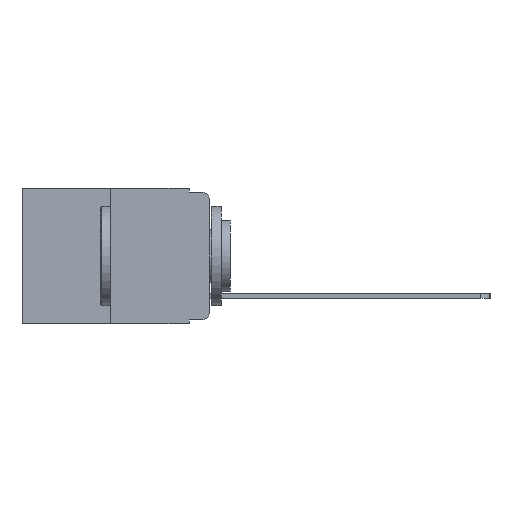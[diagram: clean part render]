
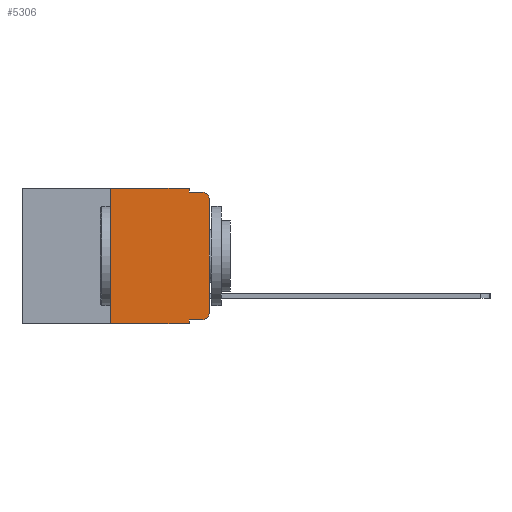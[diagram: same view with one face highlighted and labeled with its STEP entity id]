
A CAD part, left-side view. The second image highlights one B-rep face of the part: STEP entity #5306.
In plain terms, the highlighted planar face has unit normal (-1, 0, 0).
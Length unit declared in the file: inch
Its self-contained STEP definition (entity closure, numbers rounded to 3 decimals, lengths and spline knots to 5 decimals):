
#156 = CARTESIAN_POINT ( 'NONE',  ( 0., 0.051, 0. ) ) ;
#207 = VECTOR ( 'NONE', #7608, 39.37008 ) ;
#285 = CARTESIAN_POINT ( 'NONE',  ( 0., 0., 0. ) ) ;
#701 = CARTESIAN_POINT ( 'NONE',  ( 0., 0.051, -0.333 ) ) ;
#1088 = EDGE_CURVE ( 'NONE', #9467, #4476, #3043, .T. ) ;
#1211 = CARTESIAN_POINT ( 'NONE',  ( 0., 0.02, -0.01 ) ) ;
#1684 = CARTESIAN_POINT ( 'NONE',  ( 0., 0., -0.03 ) ) ;
#1837 = EDGE_CURVE ( 'NONE', #7003, #9919, #7429, .T. ) ;
#2026 = ORIENTED_EDGE ( 'NONE', *, *, #10799, .T. ) ;
#2175 = CARTESIAN_POINT ( 'NONE',  ( 0., 0.051, -0.01 ) ) ;
#2226 = DIRECTION ( 'NONE',  ( 0., 0., 1. ) ) ;
#2254 = DIRECTION ( 'NONE',  ( 0., 0., -1. ) ) ;
#2274 = DIRECTION ( 'NONE',  ( -1., 0., 0. ) ) ;
#2369 = VERTEX_POINT ( 'NONE', #5458 ) ;
#2558 = VECTOR ( 'NONE', #2886, 39.37008 ) ;
#2673 = LINE ( 'NONE', #2175, #9998 ) ;
#2846 = LINE ( 'NONE', #2920, #8355 ) ;
#2886 = DIRECTION ( 'NONE',  ( 0., -1., 0. ) ) ;
#2920 = CARTESIAN_POINT ( 'NONE',  ( 0., 0.051, -0.333 ) ) ;
#3043 = LINE ( 'NONE', #7490, #207 ) ;
#3110 = CARTESIAN_POINT ( 'NONE',  ( 0., 0.051, 0. ) ) ;
#3234 = EDGE_CURVE ( 'NONE', #5201, #7003, #6945, .T. ) ;
#3285 = CARTESIAN_POINT ( 'NONE',  ( 0., 0.25, 0. ) ) ;
#3453 = EDGE_CURVE ( 'NONE', #9909, #11802, #5152, .T. ) ;
#3486 = AXIS2_PLACEMENT_3D ( 'NONE', #8108, #2274, #2254 ) ;
#3503 = AXIS2_PLACEMENT_3D ( 'NONE', #9699, #10596, #6112 ) ;
#3666 = VERTEX_POINT ( 'NONE', #701 ) ;
#3677 = VERTEX_POINT ( 'NONE', #1211 ) ;
#3791 = PLANE ( 'NONE',  #3503 ) ;
#3971 = DIRECTION ( 'NONE',  ( 0., -1., 0. ) ) ;
#4102 = EDGE_LOOP ( 'NONE', ( #4177, #6776, #9177, #11504, #4493, #7070, #2026, #4822, #7376, #12063 ) ) ;
#4166 = LINE ( 'NONE', #156, #6481 ) ;
#4177 = ORIENTED_EDGE ( 'NONE', *, *, #1837, .T. ) ;
#4402 = EDGE_CURVE ( 'NONE', #9919, #3677, #12333, .T. ) ;
#4476 = VERTEX_POINT ( 'NONE', #8249 ) ;
#4493 = ORIENTED_EDGE ( 'NONE', *, *, #10351, .F. ) ;
#4822 = ORIENTED_EDGE ( 'NONE', *, *, #11854, .F. ) ;
#5036 = VECTOR ( 'NONE', #6316, 39.37008 ) ;
#5152 = LINE ( 'NONE', #10965, #9736 ) ;
#5201 = VERTEX_POINT ( 'NONE', #8906 ) ;
#5306 = ADVANCED_FACE ( 'NONE', ( #5813 ), #3791, .F. ) ;
#5458 = CARTESIAN_POINT ( 'NONE',  ( 0., 0.051, -0.343 ) ) ;
#5636 = LINE ( 'NONE', #5984, #2558 ) ;
#5813 = FACE_OUTER_BOUND ( 'NONE', #4102, .T. ) ;
#5984 = CARTESIAN_POINT ( 'NONE',  ( 0., 0.473, -0.343 ) ) ;
#6112 = DIRECTION ( 'NONE',  ( 0., 0., -1. ) ) ;
#6316 = DIRECTION ( 'NONE',  ( 0., -1., 0. ) ) ;
#6481 = VECTOR ( 'NONE', #8216, 39.37008 ) ;
#6776 = ORIENTED_EDGE ( 'NONE', *, *, #4402, .T. ) ;
#6945 = CIRCLE ( 'NONE', #3486, 0.02 ) ;
#7003 = VERTEX_POINT ( 'NONE', #7878 ) ;
#7070 = ORIENTED_EDGE ( 'NONE', *, *, #3453, .F. ) ;
#7376 = ORIENTED_EDGE ( 'NONE', *, *, #11530, .T. ) ;
#7429 = LINE ( 'NONE', #285, #9229 ) ;
#7490 = CARTESIAN_POINT ( 'NONE',  ( 0., 0.051, 0. ) ) ;
#7608 = DIRECTION ( 'NONE',  ( 0., 0., -1. ) ) ;
#7669 = CARTESIAN_POINT ( 'NONE',  ( 0., 0.25, -0.343 ) ) ;
#7878 = CARTESIAN_POINT ( 'NONE',  ( 0., 0., -0.313 ) ) ;
#8108 = CARTESIAN_POINT ( 'NONE',  ( 0., 0.02, -0.313 ) ) ;
#8216 = DIRECTION ( 'NONE',  ( 0., 0., -1. ) ) ;
#8249 = CARTESIAN_POINT ( 'NONE',  ( 0., 0.051, -0.01 ) ) ;
#8355 = VECTOR ( 'NONE', #3971, 39.37008 ) ;
#8906 = CARTESIAN_POINT ( 'NONE',  ( 0., 0.02, -0.333 ) ) ;
#9177 = ORIENTED_EDGE ( 'NONE', *, *, #11765, .F. ) ;
#9229 = VECTOR ( 'NONE', #2226, 39.37008 ) ;
#9467 = VERTEX_POINT ( 'NONE', #3110 ) ;
#9699 = CARTESIAN_POINT ( 'NONE',  ( 0., 0.473, 0. ) ) ;
#9736 = VECTOR ( 'NONE', #9876, 39.37008 ) ;
#9867 = DIRECTION ( 'NONE',  ( 0., -1., 0. ) ) ;
#9876 = DIRECTION ( 'NONE',  ( 0., 0., 1. ) ) ;
#9901 = CARTESIAN_POINT ( 'NONE',  ( 0., 0.473, 0. ) ) ;
#9909 = VERTEX_POINT ( 'NONE', #7669 ) ;
#9919 = VERTEX_POINT ( 'NONE', #1684 ) ;
#9998 = VECTOR ( 'NONE', #9867, 39.37008 ) ;
#10351 = EDGE_CURVE ( 'NONE', #11802, #9467, #12241, .T. ) ;
#10596 = DIRECTION ( 'NONE',  ( 1., 0., 0. ) ) ;
#10799 = EDGE_CURVE ( 'NONE', #9909, #2369, #5636, .T. ) ;
#10965 = CARTESIAN_POINT ( 'NONE',  ( 0., 0.25, 0. ) ) ;
#11504 = ORIENTED_EDGE ( 'NONE', *, *, #1088, .F. ) ;
#11510 = DIRECTION ( 'NONE',  ( 0., 0., -1. ) ) ;
#11525 = DIRECTION ( 'NONE',  ( -1., 0., 0. ) ) ;
#11530 = EDGE_CURVE ( 'NONE', #3666, #5201, #2846, .T. ) ;
#11540 = CARTESIAN_POINT ( 'NONE',  ( 0., 0.02, -0.03 ) ) ;
#11669 = AXIS2_PLACEMENT_3D ( 'NONE', #11540, #11525, #11510 ) ;
#11765 = EDGE_CURVE ( 'NONE', #4476, #3677, #2673, .T. ) ;
#11802 = VERTEX_POINT ( 'NONE', #3285 ) ;
#11854 = EDGE_CURVE ( 'NONE', #3666, #2369, #4166, .T. ) ;
#12063 = ORIENTED_EDGE ( 'NONE', *, *, #3234, .T. ) ;
#12241 = LINE ( 'NONE', #9901, #5036 ) ;
#12333 = CIRCLE ( 'NONE', #11669, 0.02 ) ;
